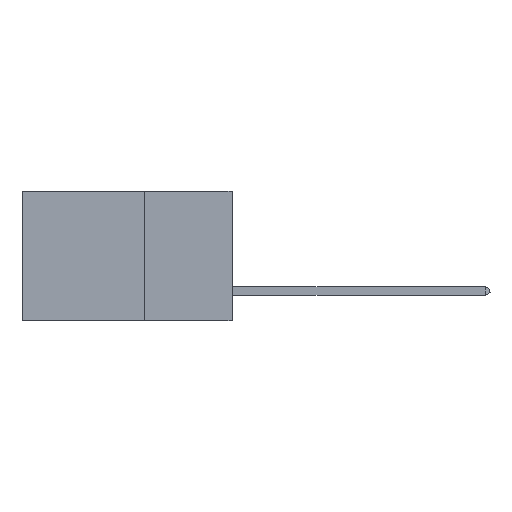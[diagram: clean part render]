
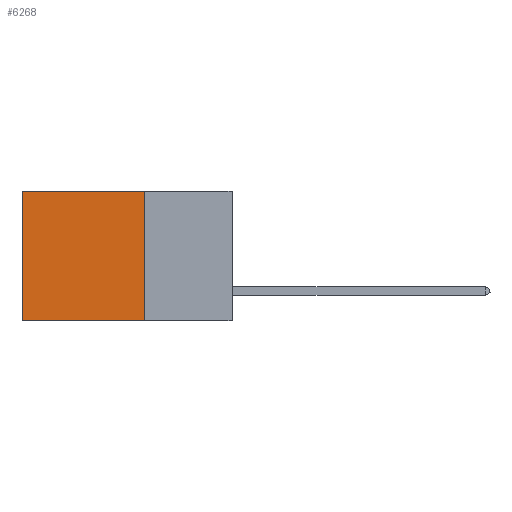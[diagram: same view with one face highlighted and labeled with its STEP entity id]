
A CAD part, left-side view. The second image highlights one B-rep face of the part: STEP entity #6268.
In plain terms, the highlighted planar face has unit normal (-1, 0, 0).
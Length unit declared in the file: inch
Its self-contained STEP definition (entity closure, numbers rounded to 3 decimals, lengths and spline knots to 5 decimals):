
#27 = VERTEX_POINT ( 'NONE', #28776 ) ;
#149 = DIRECTION ( 'NONE',  ( 0., 1., 0. ) ) ;
#1377 = CARTESIAN_POINT ( 'NONE',  ( 0.2875, 0.25, 0. ) ) ;
#1617 = CARTESIAN_POINT ( 'NONE',  ( 0.2875, 0.6, 0. ) ) ;
#1712 = DIRECTION ( 'NONE',  ( 0., 0., -1. ) ) ;
#1718 = ORIENTED_EDGE ( 'NONE', *, *, #10324, .T. ) ;
#5956 = EDGE_LOOP ( 'NONE', ( #27658, #29415, #19918, #1718 ) ) ;
#6268 = ADVANCED_FACE ( 'NONE', ( #8868 ), #10801, .F. ) ;
#7380 = CARTESIAN_POINT ( 'NONE',  ( 0.2875, 0.25, -0.37 ) ) ;
#7511 = VECTOR ( 'NONE', #149, 39.37008 ) ;
#8193 = EDGE_CURVE ( 'NONE', #25872, #9619, #17642, .T. ) ;
#8868 = FACE_OUTER_BOUND ( 'NONE', #5956, .T. ) ;
#8913 = EDGE_CURVE ( 'NONE', #27, #25872, #9804, .T. ) ;
#9072 = CARTESIAN_POINT ( 'NONE',  ( 0.2875, 0.6, -0.37 ) ) ;
#9240 = DIRECTION ( 'NONE',  ( 0., 0., -1. ) ) ;
#9619 = VERTEX_POINT ( 'NONE', #9072 ) ;
#9804 = LINE ( 'NONE', #1377, #10169 ) ;
#10169 = VECTOR ( 'NONE', #1712, 39.37008 ) ;
#10324 = EDGE_CURVE ( 'NONE', #27, #12515, #18724, .T. ) ;
#10605 = CARTESIAN_POINT ( 'NONE',  ( 0.2875, 0.25, -0.37 ) ) ;
#10757 = AXIS2_PLACEMENT_3D ( 'NONE', #15946, #30823, #11103 ) ;
#10801 = PLANE ( 'NONE',  #10757 ) ;
#11103 = DIRECTION ( 'NONE',  ( 0., 0., -1. ) ) ;
#12111 = VECTOR ( 'NONE', #30601, 39.37008 ) ;
#12515 = VERTEX_POINT ( 'NONE', #13231 ) ;
#13210 = CARTESIAN_POINT ( 'NONE',  ( 0.2875, 0.25, 0. ) ) ;
#13231 = CARTESIAN_POINT ( 'NONE',  ( 0.2875, 0.6, 0. ) ) ;
#14090 = EDGE_CURVE ( 'NONE', #12515, #9619, #27064, .T. ) ;
#15946 = CARTESIAN_POINT ( 'NONE',  ( 0.2875, 0.25, 0. ) ) ;
#17642 = LINE ( 'NONE', #7380, #7511 ) ;
#18724 = LINE ( 'NONE', #13210, #12111 ) ;
#19668 = VECTOR ( 'NONE', #9240, 39.37008 ) ;
#19918 = ORIENTED_EDGE ( 'NONE', *, *, #8913, .F. ) ;
#25872 = VERTEX_POINT ( 'NONE', #10605 ) ;
#27064 = LINE ( 'NONE', #1617, #19668 ) ;
#27658 = ORIENTED_EDGE ( 'NONE', *, *, #14090, .T. ) ;
#28776 = CARTESIAN_POINT ( 'NONE',  ( 0.2875, 0.25, 0. ) ) ;
#29415 = ORIENTED_EDGE ( 'NONE', *, *, #8193, .F. ) ;
#30601 = DIRECTION ( 'NONE',  ( 0., 1., 0. ) ) ;
#30823 = DIRECTION ( 'NONE',  ( 1., 0., 0. ) ) ;
